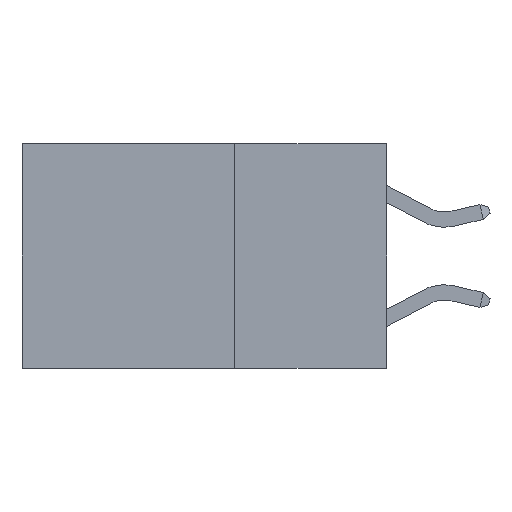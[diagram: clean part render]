
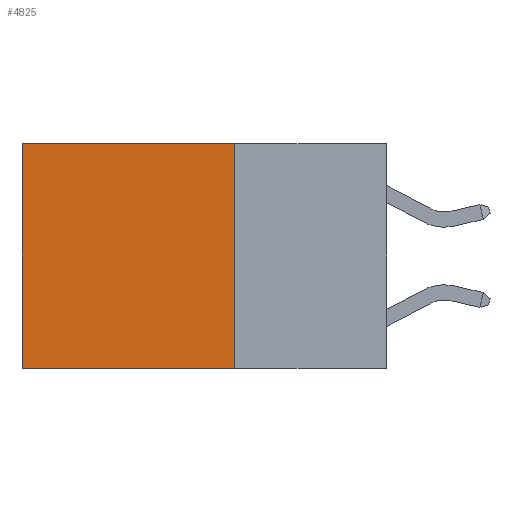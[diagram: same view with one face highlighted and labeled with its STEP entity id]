
A CAD part, left-side view. The second image highlights one B-rep face of the part: STEP entity #4825.
In plain terms, the highlighted planar face has unit normal (-1, 0, 0).
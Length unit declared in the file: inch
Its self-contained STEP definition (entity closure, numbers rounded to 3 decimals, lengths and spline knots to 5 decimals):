
#102 = FACE_OUTER_BOUND ( 'NONE', #3608, .T. ) ;
#575 = ORIENTED_EDGE ( 'NONE', *, *, #2010, .F. ) ;
#1359 = LINE ( 'NONE', #11275, #2582 ) ;
#1898 = DIRECTION ( 'NONE',  ( 0., 0., -1. ) ) ;
#2010 = EDGE_CURVE ( 'NONE', #5898, #6288, #1359, .T. ) ;
#2145 = AXIS2_PLACEMENT_3D ( 'NONE', #6992, #11035, #1898 ) ;
#2424 = DIRECTION ( 'NONE',  ( 0., 0., -1. ) ) ;
#2582 = VECTOR ( 'NONE', #2424, 39.37008 ) ;
#3608 = EDGE_LOOP ( 'NONE', ( #11130, #8328, #575, #12957 ) ) ;
#3909 = PLANE ( 'NONE',  #2145 ) ;
#4291 = DIRECTION ( 'NONE',  ( 0., 1., 0. ) ) ;
#4448 = LINE ( 'NONE', #5387, #9065 ) ;
#4551 = VERTEX_POINT ( 'NONE', #5051 ) ;
#4762 = CARTESIAN_POINT ( 'NONE',  ( 0.2625, 0.6, 0. ) ) ;
#4825 = ADVANCED_FACE ( 'NONE', ( #102 ), #3909, .F. ) ;
#4962 = DIRECTION ( 'NONE',  ( 0., 0., -1. ) ) ;
#5051 = CARTESIAN_POINT ( 'NONE',  ( 0.2625, 0.6, 0. ) ) ;
#5263 = CARTESIAN_POINT ( 'NONE',  ( 0.2625, 0.25, -0.37 ) ) ;
#5316 = CARTESIAN_POINT ( 'NONE',  ( 0.2625, 0.25, -0.37 ) ) ;
#5387 = CARTESIAN_POINT ( 'NONE',  ( 0.2625, 0.25, 0. ) ) ;
#5584 = EDGE_CURVE ( 'NONE', #4551, #8508, #7743, .T. ) ;
#5898 = VERTEX_POINT ( 'NONE', #12133 ) ;
#5924 = VECTOR ( 'NONE', #4962, 39.37008 ) ;
#6284 = LINE ( 'NONE', #5316, #11515 ) ;
#6288 = VERTEX_POINT ( 'NONE', #5263 ) ;
#6992 = CARTESIAN_POINT ( 'NONE',  ( 0.2625, 0.25, 0. ) ) ;
#7569 = EDGE_CURVE ( 'NONE', #5898, #4551, #4448, .T. ) ;
#7743 = LINE ( 'NONE', #4762, #5924 ) ;
#8328 = ORIENTED_EDGE ( 'NONE', *, *, #10619, .F. ) ;
#8508 = VERTEX_POINT ( 'NONE', #11317 ) ;
#9065 = VECTOR ( 'NONE', #11423, 39.37008 ) ;
#10619 = EDGE_CURVE ( 'NONE', #6288, #8508, #6284, .T. ) ;
#11035 = DIRECTION ( 'NONE',  ( 1., 0., 0. ) ) ;
#11130 = ORIENTED_EDGE ( 'NONE', *, *, #5584, .T. ) ;
#11275 = CARTESIAN_POINT ( 'NONE',  ( 0.2625, 0.25, 0. ) ) ;
#11317 = CARTESIAN_POINT ( 'NONE',  ( 0.2625, 0.6, -0.37 ) ) ;
#11423 = DIRECTION ( 'NONE',  ( 0., 1., 0. ) ) ;
#11515 = VECTOR ( 'NONE', #4291, 39.37008 ) ;
#12133 = CARTESIAN_POINT ( 'NONE',  ( 0.2625, 0.25, 0. ) ) ;
#12957 = ORIENTED_EDGE ( 'NONE', *, *, #7569, .T. ) ;
